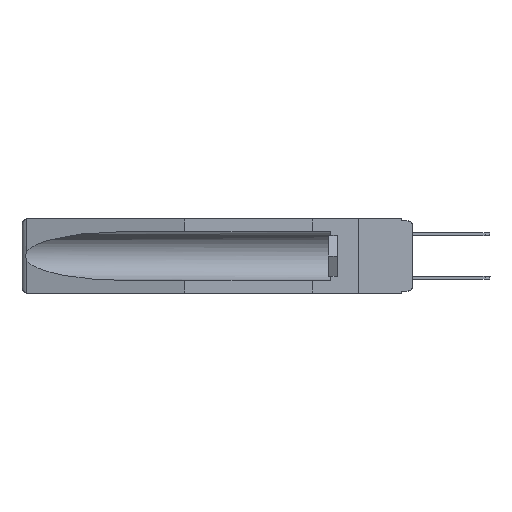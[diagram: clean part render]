
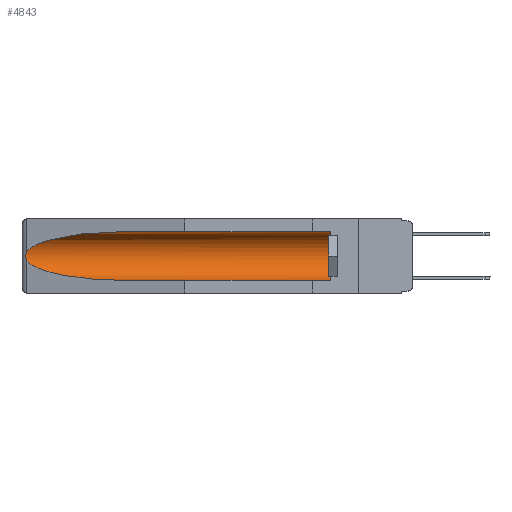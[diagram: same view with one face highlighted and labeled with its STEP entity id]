
A CAD part, left-side view. The second image highlights one B-rep face of the part: STEP entity #4843.
In plain terms, the highlighted cylindrical face has radius 2.857 mm (diameter 5.715 mm), a partial arc.
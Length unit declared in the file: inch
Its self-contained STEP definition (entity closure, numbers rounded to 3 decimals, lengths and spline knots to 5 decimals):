
#340 = DIRECTION ( 'NONE',  ( 0., 0., 1. ) ) ;
#431 = AXIS2_PLACEMENT_3D ( 'NONE', #8254, #1546, #10910 ) ;
#761 = CARTESIAN_POINT ( 'NONE',  ( 0.21114, 1.30732, -0.284 ) ) ;
#1423 = CARTESIAN_POINT ( 'NONE',  ( 0.25451, 1.48313, -0.09465 ) ) ;
#1546 = DIRECTION ( 'NONE',  ( 0., -1., 0. ) ) ;
#1599 = EDGE_CURVE ( 'NONE', #16513, #4097, #5900, .T. ) ;
#1702 = FACE_OUTER_BOUND ( 'NONE', #12686, .T. ) ;
#2545 = CARTESIAN_POINT ( 'NONE',  ( 0.26537, 1.52718, -0.19328 ) ) ;
#2903 = DIRECTION ( 'NONE',  ( 0., 1., 0. ) ) ;
#3138 = CARTESIAN_POINT ( 'NONE',  ( 0.155, 0.126, -0.059 ) ) ;
#3628 = CARTESIAN_POINT ( 'NONE',  ( 0.26655, 1.53094, -0.18657 ) ) ;
#3767 = EDGE_CURVE ( 'NONE', #14881, #6509, #11628, .T. ) ;
#4097 = VERTEX_POINT ( 'NONE', #15185 ) ;
#4525 =( BOUNDED_CURVE ( )  B_SPLINE_CURVE ( 3, ( #12616, #11415, #761, #7578 ),
 .UNSPECIFIED., .F., .T. ) 
 B_SPLINE_CURVE_WITH_KNOTS ( ( 4, 4 ),
 ( 0.1948, 1.5708 ),
 .UNSPECIFIED. ) 
 CURVE ( )  GEOMETRIC_REPRESENTATION_ITEM ( )  RATIONAL_B_SPLINE_CURVE ( ( 1., 0.848, 0.848, 1. ) ) 
 REPRESENTATION_ITEM ( '' )  );
#4843 = ADVANCED_FACE ( 'NONE', ( #1702 ), #13451, .F. ) ;
#4986 = CARTESIAN_POINT ( 'NONE',  ( 0.155, -0.30754, -0.059 ) ) ;
#5064 = CIRCLE ( 'NONE', #431, 0.1125 ) ;
#5253 = CARTESIAN_POINT ( 'NONE',  ( 0.26537, 1.52718, -0.14972 ) ) ;
#5297 = EDGE_CURVE ( 'NONE', #10335, #14881, #12706, .T. ) ;
#5334 = ORIENTED_EDGE ( 'NONE', *, *, #1599, .F. ) ;
#5633 = CARTESIAN_POINT ( 'NONE',  ( 0.155, 0.126, -0.284 ) ) ;
#5900 = LINE ( 'NONE', #12559, #12779 ) ;
#6285 = CARTESIAN_POINT ( 'NONE',  ( 0.2673, 1.5327, -0.16383 ) ) ;
#6509 = VERTEX_POINT ( 'NONE', #15750 ) ;
#6544 = ORIENTED_EDGE ( 'NONE', *, *, #13290, .T. ) ;
#7578 = CARTESIAN_POINT ( 'NONE',  ( 0.155, 1.07973, -0.284 ) ) ;
#7700 = EDGE_CURVE ( 'NONE', #6509, #4097, #4525, .T. ) ;
#7819 = CARTESIAN_POINT ( 'NONE',  ( 0.2675, 1.53308, -0.17534 ) ) ;
#8254 = CARTESIAN_POINT ( 'NONE',  ( 0.155, 0.126, -0.1715 ) ) ;
#8632 = DIRECTION ( 'NONE',  ( 0., 1., 0. ) ) ;
#8923 = CARTESIAN_POINT ( 'NONE',  ( 0.26597, 1.52961, -0.15275 ) ) ;
#9166 = CARTESIAN_POINT ( 'NONE',  ( 0.155, 1.07973, -0.059 ) ) ;
#10191 = CARTESIAN_POINT ( 'NONE',  ( 0.26654, 1.53092, -0.15636 ) ) ;
#10225 = ORIENTED_EDGE ( 'NONE', *, *, #3767, .T. ) ;
#10335 = VERTEX_POINT ( 'NONE', #16382 ) ;
#10461 = CARTESIAN_POINT ( 'NONE',  ( 0.2673, 1.53269, -0.17917 ) ) ;
#10623 = ORIENTED_EDGE ( 'NONE', *, *, #7700, .T. ) ;
#10864 = ORIENTED_EDGE ( 'NONE', *, *, #12416, .T. ) ;
#10910 = DIRECTION ( 'NONE',  ( 0., 0., 1. ) ) ;
#11304 = VERTEX_POINT ( 'NONE', #3138 ) ;
#11415 = CARTESIAN_POINT ( 'NONE',  ( 0.25451, 1.48313, -0.24835 ) ) ;
#11525 = CARTESIAN_POINT ( 'NONE',  ( 0.26537, 1.52718, -0.14972 ) ) ;
#11628 = B_SPLINE_CURVE_WITH_KNOTS ( 'NONE', 3,
 ( #5253, #8923, #10191, #6285, #14210, #7819, #10461, #3628, #12934, #2545 ),
 .UNSPECIFIED., .F., .F.,
 ( 4, 2, 2, 2, 4 ),
 ( 0., 0.00029, 0.00058, 0.00087, 0.00117 ),
 .UNSPECIFIED. ) ;
#11820 = CARTESIAN_POINT ( 'NONE',  ( 0.26537, 1.52718, -0.14972 ) ) ;
#12416 = EDGE_CURVE ( 'NONE', #16513, #11304, #5064, .T. ) ;
#12559 = CARTESIAN_POINT ( 'NONE',  ( 0.155, -0.30754, -0.284 ) ) ;
#12616 = CARTESIAN_POINT ( 'NONE',  ( 0.26537, 1.52718, -0.19328 ) ) ;
#12686 = EDGE_LOOP ( 'NONE', ( #15271, #10225, #10623, #5334, #10864, #6544 ) ) ;
#12706 =( BOUNDED_CURVE ( )  B_SPLINE_CURVE ( 3, ( #9166, #14364, #1423, #11820 ),
 .UNSPECIFIED., .F., .T. ) 
 B_SPLINE_CURVE_WITH_KNOTS ( ( 4, 4 ),
 ( 4.71239, 6.08839 ),
 .UNSPECIFIED. ) 
 CURVE ( )  GEOMETRIC_REPRESENTATION_ITEM ( )  RATIONAL_B_SPLINE_CURVE ( ( 1., 0.848, 0.848, 1. ) ) 
 REPRESENTATION_ITEM ( '' )  );
#12779 = VECTOR ( 'NONE', #8632, 39.37008 ) ;
#12934 = CARTESIAN_POINT ( 'NONE',  ( 0.26597, 1.5296, -0.19026 ) ) ;
#13290 = EDGE_CURVE ( 'NONE', #11304, #10335, #16739, .T. ) ;
#13451 = CYLINDRICAL_SURFACE ( 'NONE', #16661, 0.1125 ) ;
#14028 = VECTOR ( 'NONE', #15385, 39.37008 ) ;
#14210 = CARTESIAN_POINT ( 'NONE',  ( 0.2675, 1.53308, -0.16763 ) ) ;
#14364 = CARTESIAN_POINT ( 'NONE',  ( 0.21114, 1.30732, -0.059 ) ) ;
#14881 = VERTEX_POINT ( 'NONE', #11525 ) ;
#15185 = CARTESIAN_POINT ( 'NONE',  ( 0.155, 1.07973, -0.284 ) ) ;
#15271 = ORIENTED_EDGE ( 'NONE', *, *, #5297, .T. ) ;
#15385 = DIRECTION ( 'NONE',  ( 0., 1., 0. ) ) ;
#15750 = CARTESIAN_POINT ( 'NONE',  ( 0.26537, 1.52718, -0.19328 ) ) ;
#15921 = CARTESIAN_POINT ( 'NONE',  ( 0.155, -0.30754, -0.1715 ) ) ;
#16382 = CARTESIAN_POINT ( 'NONE',  ( 0.155, 1.07973, -0.059 ) ) ;
#16513 = VERTEX_POINT ( 'NONE', #5633 ) ;
#16661 = AXIS2_PLACEMENT_3D ( 'NONE', #15921, #2903, #340 ) ;
#16739 = LINE ( 'NONE', #4986, #14028 ) ;
